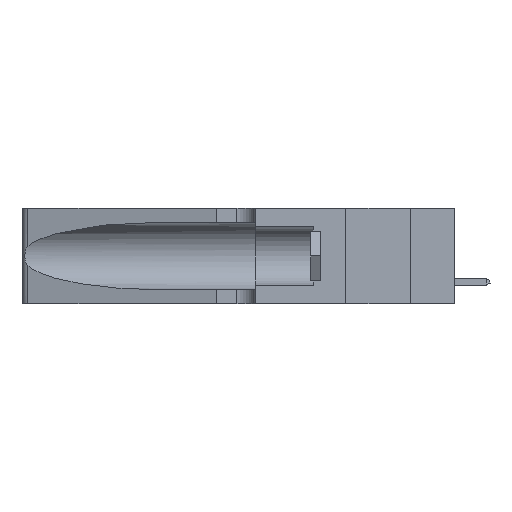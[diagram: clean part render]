
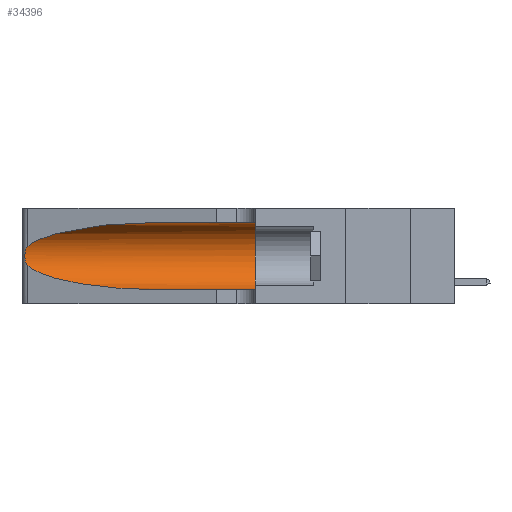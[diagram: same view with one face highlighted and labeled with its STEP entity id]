
A CAD part, left-side view. The second image highlights one B-rep face of the part: STEP entity #34396.
In plain terms, the highlighted cylindrical face has radius 3.308 mm (diameter 6.617 mm), a partial arc.
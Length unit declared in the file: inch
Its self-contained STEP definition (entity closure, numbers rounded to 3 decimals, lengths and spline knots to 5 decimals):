
#229 = CARTESIAN_POINT ( 'NONE',  ( 0.25856, 1.23593, 0.16098 ) ) ;
#303 = VECTOR ( 'NONE', #37519, 39.37008 ) ;
#324 = CYLINDRICAL_SURFACE ( 'NONE', #29400, 0.13025 ) ;
#1530 = DIRECTION ( 'NONE',  ( 0., 0., 1. ) ) ;
#1965 = CARTESIAN_POINT ( 'NONE',  ( 0.1305, 0.35, 0.185 ) ) ;
#3663 = CARTESIAN_POINT ( 'NONE',  ( 0.2373, 1.15595, 0.08982 ) ) ;
#3785 = FACE_OUTER_BOUND ( 'NONE', #31912, .T. ) ;
#3900 = VECTOR ( 'NONE', #17027, 39.37008 ) ;
#5358 = DIRECTION ( 'NONE',  ( 0., 0., -1. ) ) ;
#6356 = ORIENTED_EDGE ( 'NONE', *, *, #23001, .T. ) ;
#6630 = CARTESIAN_POINT ( 'NONE',  ( 0.25555, 1.22993, 0.14849 ) ) ;
#6876 = CARTESIAN_POINT ( 'NONE',  ( 0.25639, 1.23186, 0.15144 ) ) ;
#7053 = CARTESIAN_POINT ( 'NONE',  ( 0.1305, 0.35, 0.05475 ) ) ;
#10797 = ORIENTED_EDGE ( 'NONE', *, *, #33167, .F. ) ;
#10807 = CARTESIAN_POINT ( 'NONE',  ( 0.1305, 1.61858, 0.185 ) ) ;
#12076 = CARTESIAN_POINT ( 'NONE',  ( 0.1305, 0.72297, 0.31525 ) ) ;
#12493 = CARTESIAN_POINT ( 'NONE',  ( 0.1305, 1.61858, 0.05475 ) ) ;
#12624 =( BOUNDED_CURVE ( )  B_SPLINE_CURVE ( 3, ( #22804, #3663, #29200, #19420 ),
 .UNSPECIFIED., .F., .T. ) 
 B_SPLINE_CURVE_WITH_KNOTS ( ( 4, 4 ),
 ( 3.44316, 4.71239 ),
 .UNSPECIFIED. ) 
 CURVE ( )  GEOMETRIC_REPRESENTATION_ITEM ( )  RATIONAL_B_SPLINE_CURVE ( ( 1., 0.87, 0.87, 1. ) ) 
 REPRESENTATION_ITEM ( '' )  );
#12750 = CARTESIAN_POINT ( 'NONE',  ( 0.26018, 1.23835, 0.19895 ) ) ;
#14230 = DIRECTION ( 'NONE',  ( 0., -1., 0. ) ) ;
#15200 = VERTEX_POINT ( 'NONE', #7053 ) ;
#15527 = VERTEX_POINT ( 'NONE', #16512 ) ;
#15973 = CARTESIAN_POINT ( 'NONE',  ( 0.25787, 1.23484, 0.2124 ) ) ;
#16105 = CARTESIAN_POINT ( 'NONE',  ( 0.25639, 1.23184, 0.21858 ) ) ;
#16512 = CARTESIAN_POINT ( 'NONE',  ( 0.25487, 1.22718, 0.14631 ) ) ;
#16944 =( BOUNDED_CURVE ( )  B_SPLINE_CURVE ( 3, ( #12076, #30812, #30943, #18503 ),
 .UNSPECIFIED., .F., .T. ) 
 B_SPLINE_CURVE_WITH_KNOTS ( ( 4, 4 ),
 ( 1.5708, 2.84003 ),
 .UNSPECIFIED. ) 
 CURVE ( )  GEOMETRIC_REPRESENTATION_ITEM ( )  RATIONAL_B_SPLINE_CURVE ( ( 1., 0.87, 0.87, 1. ) ) 
 REPRESENTATION_ITEM ( '' )  );
#17027 = DIRECTION ( 'NONE',  ( 0., -1., 0. ) ) ;
#17238 = VERTEX_POINT ( 'NONE', #30202 ) ;
#17324 = ORIENTED_EDGE ( 'NONE', *, *, #37953, .T. ) ;
#17702 = CARTESIAN_POINT ( 'NONE',  ( 0.1305, 0.72297, 0.31525 ) ) ;
#17947 = VERTEX_POINT ( 'NONE', #17702 ) ;
#18451 = ORIENTED_EDGE ( 'NONE', *, *, #41031, .T. ) ;
#18503 = CARTESIAN_POINT ( 'NONE',  ( 0.25487, 1.22718, 0.22369 ) ) ;
#19320 = CARTESIAN_POINT ( 'NONE',  ( 0.26075, 1.23896, 0.178 ) ) ;
#19420 = CARTESIAN_POINT ( 'NONE',  ( 0.1305, 0.72297, 0.05475 ) ) ;
#19603 = CARTESIAN_POINT ( 'NONE',  ( 0.26017, 1.23833, 0.17102 ) ) ;
#21974 = LINE ( 'NONE', #23085, #3900 ) ;
#22437 = CARTESIAN_POINT ( 'NONE',  ( 0.25487, 1.22718, 0.14631 ) ) ;
#22804 = CARTESIAN_POINT ( 'NONE',  ( 0.25487, 1.22718, 0.14631 ) ) ;
#23001 = EDGE_CURVE ( 'NONE', #24062, #15200, #37793, .T. ) ;
#23085 = CARTESIAN_POINT ( 'NONE',  ( 0.1305, 1.61858, 0.31525 ) ) ;
#23433 = CIRCLE ( 'NONE', #36046, 0.13025 ) ;
#24062 = VERTEX_POINT ( 'NONE', #31674 ) ;
#24987 = CARTESIAN_POINT ( 'NONE',  ( 0.1305, 0.35, 0.31525 ) ) ;
#25567 = ORIENTED_EDGE ( 'NONE', *, *, #39936, .T. ) ;
#25664 = CARTESIAN_POINT ( 'NONE',  ( 0.26075, 1.23896, 0.19203 ) ) ;
#28116 = EDGE_CURVE ( 'NONE', #17947, #39254, #21974, .T. ) ;
#28693 = CARTESIAN_POINT ( 'NONE',  ( 0.25487, 1.22718, 0.22369 ) ) ;
#29200 = CARTESIAN_POINT ( 'NONE',  ( 0.18966, 0.96281, 0.05475 ) ) ;
#29400 = AXIS2_PLACEMENT_3D ( 'NONE', #10807, #14230, #5358 ) ;
#30202 = CARTESIAN_POINT ( 'NONE',  ( 0.25487, 1.22718, 0.22369 ) ) ;
#30812 = CARTESIAN_POINT ( 'NONE',  ( 0.18966, 0.96281, 0.31525 ) ) ;
#30943 = CARTESIAN_POINT ( 'NONE',  ( 0.2373, 1.15595, 0.28018 ) ) ;
#31674 = CARTESIAN_POINT ( 'NONE',  ( 0.1305, 0.72297, 0.05475 ) ) ;
#31912 = EDGE_LOOP ( 'NONE', ( #17324, #18451, #25567, #6356, #10797, #34659 ) ) ;
#33112 = B_SPLINE_CURVE_WITH_KNOTS ( 'NONE', 3,
 ( #28693, #38742, #16105, #15973, #38467, #12750, #25664, #19320, #19603, #229, #38344, #6876, #6630, #22437 ),
 .UNSPECIFIED., .F., .F.,
 ( 4, 2, 2, 2, 2, 2, 4 ),
 ( 0., 0.00027, 0.00053, 0.00107, 0.0016, 0.00187, 0.00214 ),
 .UNSPECIFIED. ) ;
#33167 = EDGE_CURVE ( 'NONE', #39254, #15200, #23433, .T. ) ;
#33620 = DIRECTION ( 'NONE',  ( 0., 1., 0. ) ) ;
#34396 = ADVANCED_FACE ( 'NONE', ( #3785 ), #324, .F. ) ;
#34659 = ORIENTED_EDGE ( 'NONE', *, *, #28116, .F. ) ;
#36046 = AXIS2_PLACEMENT_3D ( 'NONE', #1965, #33620, #1530 ) ;
#37519 = DIRECTION ( 'NONE',  ( 0., -1., 0. ) ) ;
#37793 = LINE ( 'NONE', #12493, #303 ) ;
#37953 = EDGE_CURVE ( 'NONE', #17947, #17238, #16944, .T. ) ;
#38344 = CARTESIAN_POINT ( 'NONE',  ( 0.25789, 1.23486, 0.15765 ) ) ;
#38467 = CARTESIAN_POINT ( 'NONE',  ( 0.25854, 1.2359, 0.20912 ) ) ;
#38742 = CARTESIAN_POINT ( 'NONE',  ( 0.25555, 1.22994, 0.2215 ) ) ;
#39254 = VERTEX_POINT ( 'NONE', #24987 ) ;
#39936 = EDGE_CURVE ( 'NONE', #15527, #24062, #12624, .T. ) ;
#41031 = EDGE_CURVE ( 'NONE', #17238, #15527, #33112, .T. ) ;
